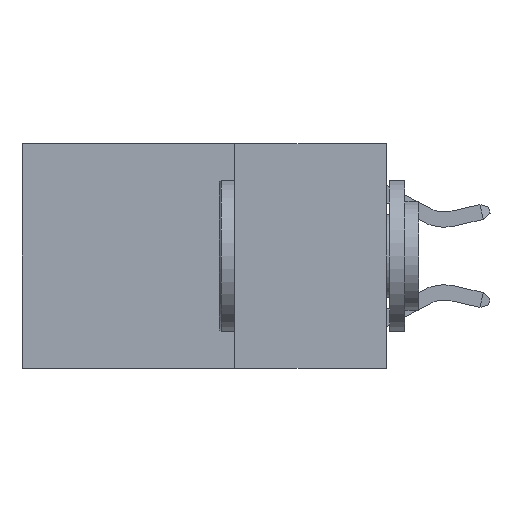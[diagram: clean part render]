
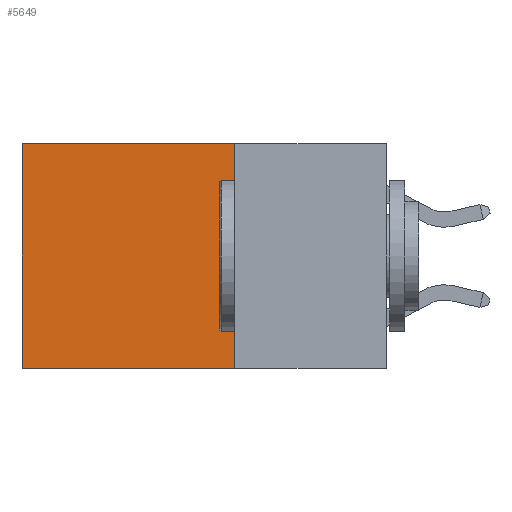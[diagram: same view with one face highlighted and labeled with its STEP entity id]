
A CAD part, left-side view. The second image highlights one B-rep face of the part: STEP entity #5649.
In plain terms, the highlighted planar face has unit normal (-1, 0, 0).
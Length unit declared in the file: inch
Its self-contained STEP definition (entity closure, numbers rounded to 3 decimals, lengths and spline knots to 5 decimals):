
#544 = CARTESIAN_POINT ( 'NONE',  ( 0.2625, 0.25, -0.37 ) ) ;
#1037 = VECTOR ( 'NONE', #9182, 39.37008 ) ;
#1324 = FACE_OUTER_BOUND ( 'NONE', #15533, .T. ) ;
#1625 = CARTESIAN_POINT ( 'NONE',  ( 0.2625, 0.6, 0. ) ) ;
#1931 = CARTESIAN_POINT ( 'NONE',  ( 0.2625, 0.6, 0. ) ) ;
#3545 = DIRECTION ( 'NONE',  ( 0., 0., -1. ) ) ;
#3605 = ORIENTED_EDGE ( 'NONE', *, *, #12846, .F. ) ;
#4327 = VERTEX_POINT ( 'NONE', #544 ) ;
#5135 = VERTEX_POINT ( 'NONE', #16137 ) ;
#5380 = VERTEX_POINT ( 'NONE', #1625 ) ;
#5383 = VECTOR ( 'NONE', #8462, 39.37008 ) ;
#5447 = DIRECTION ( 'NONE',  ( 0., 1., 0. ) ) ;
#5644 = VECTOR ( 'NONE', #5447, 39.37008 ) ;
#5649 = ADVANCED_FACE ( 'NONE', ( #1324 ), #17602, .F. ) ;
#6123 = VECTOR ( 'NONE', #3545, 39.37008 ) ;
#6337 = ORIENTED_EDGE ( 'NONE', *, *, #15223, .T. ) ;
#6512 = VERTEX_POINT ( 'NONE', #19073 ) ;
#6889 = CARTESIAN_POINT ( 'NONE',  ( 0.2625, 0.25, 0. ) ) ;
#7075 = AXIS2_PLACEMENT_3D ( 'NONE', #13304, #19053, #10458 ) ;
#7809 = ORIENTED_EDGE ( 'NONE', *, *, #14271, .F. ) ;
#8073 = EDGE_CURVE ( 'NONE', #6512, #5380, #17906, .T. ) ;
#8462 = DIRECTION ( 'NONE',  ( 0., 0., -1. ) ) ;
#9182 = DIRECTION ( 'NONE',  ( 0., 1., 0. ) ) ;
#9577 = LINE ( 'NONE', #6889, #5383 ) ;
#10458 = DIRECTION ( 'NONE',  ( 0., 0., -1. ) ) ;
#10609 = CARTESIAN_POINT ( 'NONE',  ( 0.2625, 0.25, -0.37 ) ) ;
#12846 = EDGE_CURVE ( 'NONE', #4327, #5135, #12863, .T. ) ;
#12863 = LINE ( 'NONE', #10609, #1037 ) ;
#13010 = CARTESIAN_POINT ( 'NONE',  ( 0.2625, 0.25, 0. ) ) ;
#13304 = CARTESIAN_POINT ( 'NONE',  ( 0.2625, 0.25, 0. ) ) ;
#14271 = EDGE_CURVE ( 'NONE', #6512, #4327, #9577, .T. ) ;
#15223 = EDGE_CURVE ( 'NONE', #5380, #5135, #17873, .T. ) ;
#15533 = EDGE_LOOP ( 'NONE', ( #6337, #3605, #7809, #16957 ) ) ;
#16137 = CARTESIAN_POINT ( 'NONE',  ( 0.2625, 0.6, -0.37 ) ) ;
#16957 = ORIENTED_EDGE ( 'NONE', *, *, #8073, .T. ) ;
#17602 = PLANE ( 'NONE',  #7075 ) ;
#17873 = LINE ( 'NONE', #1931, #6123 ) ;
#17906 = LINE ( 'NONE', #13010, #5644 ) ;
#19053 = DIRECTION ( 'NONE',  ( 1., 0., 0. ) ) ;
#19073 = CARTESIAN_POINT ( 'NONE',  ( 0.2625, 0.25, 0. ) ) ;
